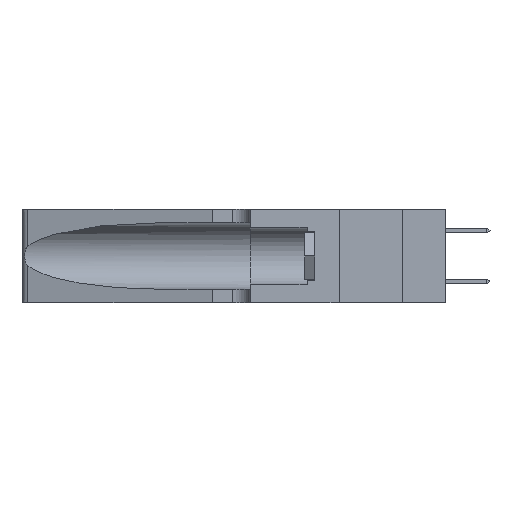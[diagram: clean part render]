
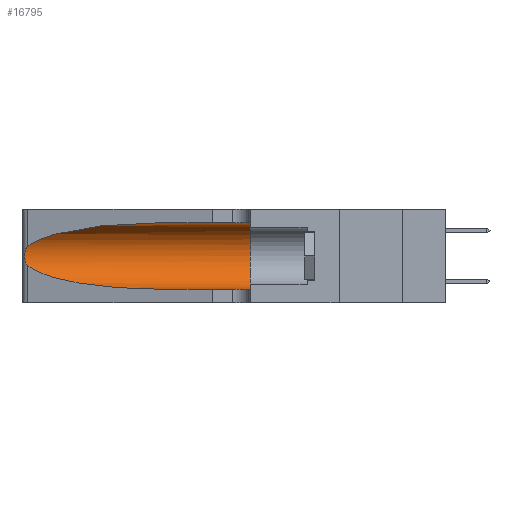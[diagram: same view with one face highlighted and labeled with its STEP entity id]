
A CAD part, left-side view. The second image highlights one B-rep face of the part: STEP entity #16795.
In plain terms, the highlighted cylindrical face has radius 3.308 mm (diameter 6.617 mm), a partial arc.
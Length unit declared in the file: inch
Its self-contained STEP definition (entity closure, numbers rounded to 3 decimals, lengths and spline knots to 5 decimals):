
#126 = CARTESIAN_POINT ( 'NONE',  ( 0.25487, 1.22718, 0.14631 ) ) ;
#563 = CARTESIAN_POINT ( 'NONE',  ( 0.25555, 1.22994, 0.2215 ) ) ;
#631 = CARTESIAN_POINT ( 'NONE',  ( 0.25854, 1.2359, 0.20912 ) ) ;
#693 = AXIS2_PLACEMENT_3D ( 'NONE', #9333, #15440, #5975 ) ;
#734 = CARTESIAN_POINT ( 'NONE',  ( 0.1305, 0.35, 0.185 ) ) ;
#1679 = CARTESIAN_POINT ( 'NONE',  ( 0.18966, 0.96281, 0.05475 ) ) ;
#2042 = CARTESIAN_POINT ( 'NONE',  ( 0.26018, 1.23835, 0.19895 ) ) ;
#2049 = CARTESIAN_POINT ( 'NONE',  ( 0.1305, 0.35, 0.31525 ) ) ;
#2181 = CARTESIAN_POINT ( 'NONE',  ( 0.26075, 1.23896, 0.19203 ) ) ;
#3616 = CARTESIAN_POINT ( 'NONE',  ( 0.25789, 1.23486, 0.15765 ) ) ;
#4126 = ORIENTED_EDGE ( 'NONE', *, *, #10753, .T. ) ;
#4475 = CARTESIAN_POINT ( 'NONE',  ( 0.25487, 1.22718, 0.22369 ) ) ;
#4491 =( BOUNDED_CURVE ( )  B_SPLINE_CURVE ( 3, ( #6018, #18667, #6092, #16772 ),
 .UNSPECIFIED., .F., .T. ) 
 B_SPLINE_CURVE_WITH_KNOTS ( ( 4, 4 ),
 ( 1.5708, 2.84003 ),
 .UNSPECIFIED. ) 
 CURVE ( )  GEOMETRIC_REPRESENTATION_ITEM ( )  RATIONAL_B_SPLINE_CURVE ( ( 1., 0.87, 0.87, 1. ) ) 
 REPRESENTATION_ITEM ( '' )  );
#4547 = ORIENTED_EDGE ( 'NONE', *, *, #7309, .T. ) ;
#4728 = CYLINDRICAL_SURFACE ( 'NONE', #693, 0.13025 ) ;
#5519 = VECTOR ( 'NONE', #9207, 39.37008 ) ;
#5659 = EDGE_CURVE ( 'NONE', #15610, #11936, #12999, .T. ) ;
#5975 = DIRECTION ( 'NONE',  ( 0., 0., -1. ) ) ;
#6018 = CARTESIAN_POINT ( 'NONE',  ( 0.1305, 0.72297, 0.31525 ) ) ;
#6032 = LINE ( 'NONE', #8949, #5519 ) ;
#6092 = CARTESIAN_POINT ( 'NONE',  ( 0.2373, 1.15595, 0.28018 ) ) ;
#6152 = VERTEX_POINT ( 'NONE', #4475 ) ;
#6680 = ORIENTED_EDGE ( 'NONE', *, *, #5659, .F. ) ;
#7102 = EDGE_LOOP ( 'NONE', ( #10939, #4126, #19693, #4547, #6680, #20057 ) ) ;
#7309 = EDGE_CURVE ( 'NONE', #13884, #11936, #6032, .T. ) ;
#7446 = CARTESIAN_POINT ( 'NONE',  ( 0.1305, 1.61858, 0.31525 ) ) ;
#7464 = EDGE_CURVE ( 'NONE', #14059, #13884, #8569, .T. ) ;
#7523 = DIRECTION ( 'NONE',  ( 0., -1., 0. ) ) ;
#8569 =( BOUNDED_CURVE ( )  B_SPLINE_CURVE ( 3, ( #126, #10998, #1679, #20418 ),
 .UNSPECIFIED., .F., .F. ) 
 B_SPLINE_CURVE_WITH_KNOTS ( ( 4, 4 ),
 ( 3.44316, 4.71239 ),
 .UNSPECIFIED. ) 
 CURVE ( )  GEOMETRIC_REPRESENTATION_ITEM ( )  RATIONAL_B_SPLINE_CURVE ( ( 1., 0.87, 0.87, 1. ) ) 
 REPRESENTATION_ITEM ( '' )  );
#8949 = CARTESIAN_POINT ( 'NONE',  ( 0.1305, 1.61858, 0.05475 ) ) ;
#9100 = CARTESIAN_POINT ( 'NONE',  ( 0.1305, 0.72297, 0.31525 ) ) ;
#9207 = DIRECTION ( 'NONE',  ( 0., -1., 0. ) ) ;
#9333 = CARTESIAN_POINT ( 'NONE',  ( 0.1305, 1.61858, 0.185 ) ) ;
#10299 = LINE ( 'NONE', #7446, #12991 ) ;
#10753 = EDGE_CURVE ( 'NONE', #6152, #14059, #11317, .T. ) ;
#10939 = ORIENTED_EDGE ( 'NONE', *, *, #20391, .T. ) ;
#10998 = CARTESIAN_POINT ( 'NONE',  ( 0.2373, 1.15595, 0.08982 ) ) ;
#11150 = AXIS2_PLACEMENT_3D ( 'NONE', #734, #13352, #13560 ) ;
#11317 = B_SPLINE_CURVE_WITH_KNOTS ( 'NONE', 3,
 ( #18539, #563, #16417, #17792, #631, #2042, #2181, #13243, #13101, #16339, #3616, #14701, #17998, #16276 ),
 .UNSPECIFIED., .F., .F.,
 ( 4, 2, 2, 2, 2, 2, 4 ),
 ( 0., 0.00027, 0.00053, 0.00107, 0.0016, 0.00187, 0.00214 ),
 .UNSPECIFIED. ) ;
#11936 = VERTEX_POINT ( 'NONE', #14101 ) ;
#12991 = VECTOR ( 'NONE', #7523, 39.37008 ) ;
#12999 = CIRCLE ( 'NONE', #11150, 0.13025 ) ;
#13101 = CARTESIAN_POINT ( 'NONE',  ( 0.26017, 1.23833, 0.17102 ) ) ;
#13243 = CARTESIAN_POINT ( 'NONE',  ( 0.26075, 1.23896, 0.178 ) ) ;
#13352 = DIRECTION ( 'NONE',  ( 0., 1., 0. ) ) ;
#13560 = DIRECTION ( 'NONE',  ( 0., 0., 1. ) ) ;
#13884 = VERTEX_POINT ( 'NONE', #15221 ) ;
#14059 = VERTEX_POINT ( 'NONE', #17907 ) ;
#14101 = CARTESIAN_POINT ( 'NONE',  ( 0.1305, 0.35, 0.05475 ) ) ;
#14140 = FACE_OUTER_BOUND ( 'NONE', #7102, .T. ) ;
#14701 = CARTESIAN_POINT ( 'NONE',  ( 0.25639, 1.23186, 0.15144 ) ) ;
#14793 = EDGE_CURVE ( 'NONE', #16418, #15610, #10299, .T. ) ;
#15221 = CARTESIAN_POINT ( 'NONE',  ( 0.1305, 0.72297, 0.05475 ) ) ;
#15440 = DIRECTION ( 'NONE',  ( 0., -1., 0. ) ) ;
#15610 = VERTEX_POINT ( 'NONE', #2049 ) ;
#16276 = CARTESIAN_POINT ( 'NONE',  ( 0.25487, 1.22718, 0.14631 ) ) ;
#16339 = CARTESIAN_POINT ( 'NONE',  ( 0.25856, 1.23593, 0.16098 ) ) ;
#16417 = CARTESIAN_POINT ( 'NONE',  ( 0.25639, 1.23184, 0.21858 ) ) ;
#16418 = VERTEX_POINT ( 'NONE', #9100 ) ;
#16772 = CARTESIAN_POINT ( 'NONE',  ( 0.25487, 1.22718, 0.22369 ) ) ;
#16795 = ADVANCED_FACE ( 'NONE', ( #14140 ), #4728, .F. ) ;
#17792 = CARTESIAN_POINT ( 'NONE',  ( 0.25787, 1.23484, 0.2124 ) ) ;
#17907 = CARTESIAN_POINT ( 'NONE',  ( 0.25487, 1.22718, 0.14631 ) ) ;
#17998 = CARTESIAN_POINT ( 'NONE',  ( 0.25555, 1.22993, 0.14849 ) ) ;
#18539 = CARTESIAN_POINT ( 'NONE',  ( 0.25487, 1.22718, 0.22369 ) ) ;
#18667 = CARTESIAN_POINT ( 'NONE',  ( 0.18966, 0.96281, 0.31525 ) ) ;
#19693 = ORIENTED_EDGE ( 'NONE', *, *, #7464, .T. ) ;
#20057 = ORIENTED_EDGE ( 'NONE', *, *, #14793, .F. ) ;
#20391 = EDGE_CURVE ( 'NONE', #16418, #6152, #4491, .T. ) ;
#20418 = CARTESIAN_POINT ( 'NONE',  ( 0.1305, 0.72297, 0.05475 ) ) ;
